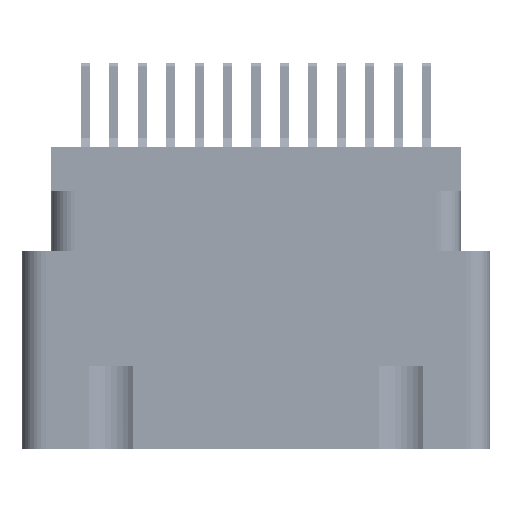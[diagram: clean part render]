
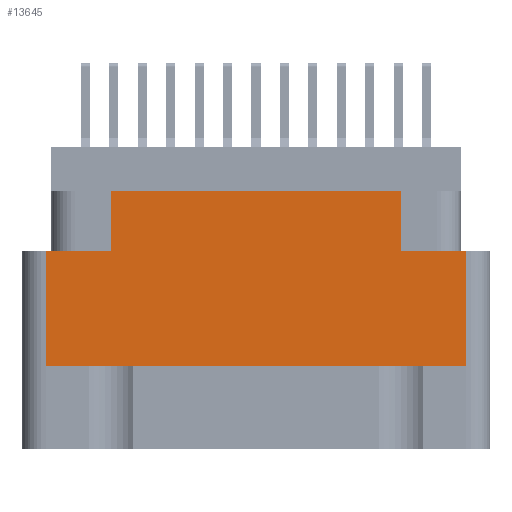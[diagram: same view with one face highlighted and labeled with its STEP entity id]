
A CAD part, left-side view. The second image highlights one B-rep face of the part: STEP entity #13645.
In plain terms, the highlighted planar face has unit normal (-1, 0, 0).
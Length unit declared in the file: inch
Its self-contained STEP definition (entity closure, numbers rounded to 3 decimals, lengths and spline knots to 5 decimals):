
#1275 = PLANE ( 'NONE',  #66710 ) ;
#2326 = VERTEX_POINT ( 'NONE', #46826 ) ;
#3569 = LINE ( 'NONE', #6164, #17521 ) ;
#5475 = ORIENTED_EDGE ( 'NONE', *, *, #54050, .T. ) ;
#6164 = CARTESIAN_POINT ( 'NONE',  ( -1.359, -0.3825, -0.274 ) ) ;
#7105 = EDGE_CURVE ( 'NONE', #7823, #2326, #59643, .T. ) ;
#7563 = FACE_OUTER_BOUND ( 'NONE', #20343, .T. ) ;
#7574 = VECTOR ( 'NONE', #11875, 39.37008 ) ;
#7823 = VERTEX_POINT ( 'NONE', #28893 ) ;
#8739 = LINE ( 'NONE', #39245, #37536 ) ;
#9159 = VERTEX_POINT ( 'NONE', #31091 ) ;
#10495 = CARTESIAN_POINT ( 'NONE',  ( -1.359, 0.3825, -0.274 ) ) ;
#10858 = LINE ( 'NONE', #55130, #60053 ) ;
#11875 = DIRECTION ( 'NONE',  ( 0., -1., 0. ) ) ;
#12593 = VERTEX_POINT ( 'NONE', #40441 ) ;
#13267 = EDGE_CURVE ( 'NONE', #55531, #53172, #3569, .T. ) ;
#13645 = ADVANCED_FACE ( 'NONE', ( #7563 ), #1275, .T. ) ;
#14828 = ORIENTED_EDGE ( 'NONE', *, *, #35683, .F. ) ;
#16850 = EDGE_CURVE ( 'NONE', #12593, #9159, #38641, .T. ) ;
#17521 = VECTOR ( 'NONE', #65054, 39.37008 ) ;
#18679 = VECTOR ( 'NONE', #28942, 39.37008 ) ;
#19086 = VERTEX_POINT ( 'NONE', #22374 ) ;
#20343 = EDGE_LOOP ( 'NONE', ( #14828, #34670, #44758, #5475, #32084, #44395, #46471, #37826 ) ) ;
#21128 = DIRECTION ( 'NONE',  ( 0., 0., 1. ) ) ;
#22374 = CARTESIAN_POINT ( 'NONE',  ( -1.359, -0.555, -0.578 ) ) ;
#26402 = CARTESIAN_POINT ( 'NONE',  ( -1.359, -0.555, -0.798 ) ) ;
#26543 = LINE ( 'NONE', #37416, #65077 ) ;
#27641 = CARTESIAN_POINT ( 'NONE',  ( -1.359, -0.617, -0.798 ) ) ;
#28222 = CARTESIAN_POINT ( 'NONE',  ( -1.359, -0.555, -0.274 ) ) ;
#28893 = CARTESIAN_POINT ( 'NONE',  ( -1.359, 0.555, -0.274 ) ) ;
#28942 = DIRECTION ( 'NONE',  ( 0., 0., -1. ) ) ;
#31091 = CARTESIAN_POINT ( 'NONE',  ( -1.359, 0.3825, -0.117 ) ) ;
#31803 = EDGE_CURVE ( 'NONE', #55531, #42497, #63323, .T. ) ;
#32084 = ORIENTED_EDGE ( 'NONE', *, *, #31803, .F. ) ;
#34670 = ORIENTED_EDGE ( 'NONE', *, *, #7105, .T. ) ;
#35683 = EDGE_CURVE ( 'NONE', #7823, #12593, #8739, .T. ) ;
#37416 = CARTESIAN_POINT ( 'NONE',  ( -1.359, 0.617, -0.117 ) ) ;
#37536 = VECTOR ( 'NONE', #44800, 39.37008 ) ;
#37826 = ORIENTED_EDGE ( 'NONE', *, *, #16850, .F. ) ;
#38641 = LINE ( 'NONE', #10495, #41849 ) ;
#39245 = CARTESIAN_POINT ( 'NONE',  ( -1.359, 0., -0.274 ) ) ;
#40441 = CARTESIAN_POINT ( 'NONE',  ( -1.359, 0.3825, -0.274 ) ) ;
#40614 = EDGE_CURVE ( 'NONE', #9159, #53172, #26543, .T. ) ;
#41849 = VECTOR ( 'NONE', #56819, 39.37008 ) ;
#42429 = CARTESIAN_POINT ( 'NONE',  ( -1.359, 0., -0.274 ) ) ;
#42497 = VERTEX_POINT ( 'NONE', #28222 ) ;
#42654 = DIRECTION ( 'NONE',  ( 0., -1., 0. ) ) ;
#44395 = ORIENTED_EDGE ( 'NONE', *, *, #13267, .T. ) ;
#44758 = ORIENTED_EDGE ( 'NONE', *, *, #67249, .T. ) ;
#44800 = DIRECTION ( 'NONE',  ( 0., -1., 0. ) ) ;
#46471 = ORIENTED_EDGE ( 'NONE', *, *, #40614, .F. ) ;
#46826 = CARTESIAN_POINT ( 'NONE',  ( -1.359, 0.555, -0.578 ) ) ;
#52787 = CARTESIAN_POINT ( 'NONE',  ( -1.359, -0.3825, -0.274 ) ) ;
#53074 = DIRECTION ( 'NONE',  ( -1., 0., 0. ) ) ;
#53172 = VERTEX_POINT ( 'NONE', #62570 ) ;
#54050 = EDGE_CURVE ( 'NONE', #19086, #42497, #60711, .T. ) ;
#55130 = CARTESIAN_POINT ( 'NONE',  ( -1.359, 0., -0.578 ) ) ;
#55531 = VERTEX_POINT ( 'NONE', #52787 ) ;
#56819 = DIRECTION ( 'NONE',  ( 0., 0., 1. ) ) ;
#58308 = VECTOR ( 'NONE', #21128, 39.37008 ) ;
#59643 = LINE ( 'NONE', #66437, #18679 ) ;
#60053 = VECTOR ( 'NONE', #65459, 39.37008 ) ;
#60711 = LINE ( 'NONE', #26402, #58308 ) ;
#62570 = CARTESIAN_POINT ( 'NONE',  ( -1.359, -0.3825, -0.117 ) ) ;
#63323 = LINE ( 'NONE', #42429, #7574 ) ;
#64282 = DIRECTION ( 'NONE',  ( 0., 0., 1. ) ) ;
#65054 = DIRECTION ( 'NONE',  ( 0., 0., 1. ) ) ;
#65077 = VECTOR ( 'NONE', #42654, 39.37008 ) ;
#65459 = DIRECTION ( 'NONE',  ( 0., -1., 0. ) ) ;
#66437 = CARTESIAN_POINT ( 'NONE',  ( -1.359, 0.555, -0.798 ) ) ;
#66710 = AXIS2_PLACEMENT_3D ( 'NONE', #27641, #53074, #64282 ) ;
#67249 = EDGE_CURVE ( 'NONE', #2326, #19086, #10858, .T. ) ;
